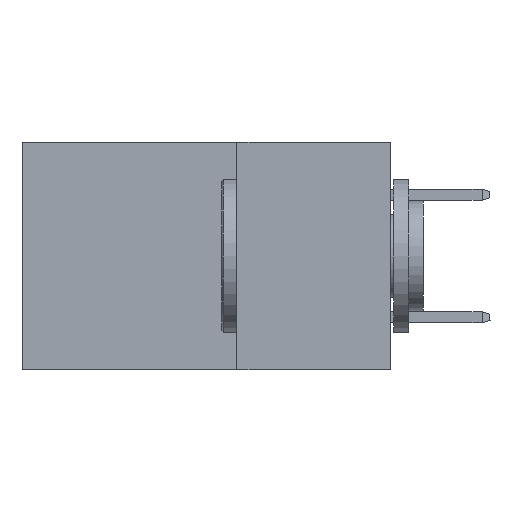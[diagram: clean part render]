
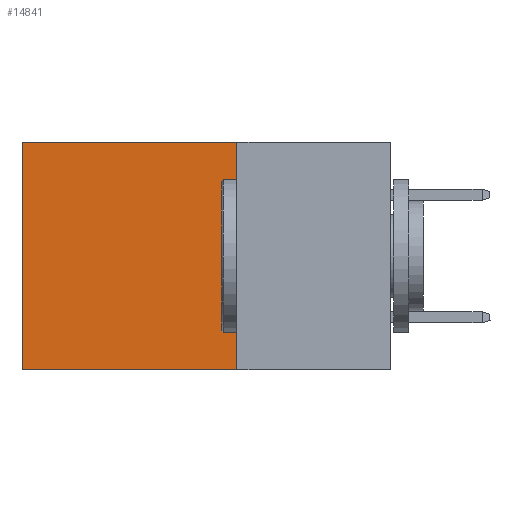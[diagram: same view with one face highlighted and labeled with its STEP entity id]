
A CAD part, left-side view. The second image highlights one B-rep face of the part: STEP entity #14841.
In plain terms, the highlighted planar face has unit normal (-1, 0, 0).
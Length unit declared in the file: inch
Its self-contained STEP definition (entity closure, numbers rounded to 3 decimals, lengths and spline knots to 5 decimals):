
#1457 = DIRECTION ( 'NONE',  ( 1., 0., 0. ) ) ;
#3225 = CARTESIAN_POINT ( 'NONE',  ( 0.2875, 0.25, -0.37 ) ) ;
#3735 = CARTESIAN_POINT ( 'NONE',  ( 0.2875, 0.25, 0. ) ) ;
#4620 = AXIS2_PLACEMENT_3D ( 'NONE', #17867, #1457, #20649 ) ;
#5412 = CARTESIAN_POINT ( 'NONE',  ( 0.2875, 0.25, 0. ) ) ;
#7098 = VERTEX_POINT ( 'NONE', #29846 ) ;
#8364 = LINE ( 'NONE', #5412, #22188 ) ;
#8397 = DIRECTION ( 'NONE',  ( 0., 0., -1. ) ) ;
#9053 = LINE ( 'NONE', #3225, #20254 ) ;
#10389 = ORIENTED_EDGE ( 'NONE', *, *, #23916, .F. ) ;
#12477 = EDGE_CURVE ( 'NONE', #31087, #7098, #18816, .T. ) ;
#14841 = ADVANCED_FACE ( 'NONE', ( #27757 ), #28886, .F. ) ;
#17867 = CARTESIAN_POINT ( 'NONE',  ( 0.2875, 0.25, 0. ) ) ;
#18354 = VERTEX_POINT ( 'NONE', #23366 ) ;
#18816 = LINE ( 'NONE', #32471, #34385 ) ;
#20254 = VECTOR ( 'NONE', #33315, 39.37008 ) ;
#20649 = DIRECTION ( 'NONE',  ( 0., 0., -1. ) ) ;
#21237 = EDGE_CURVE ( 'NONE', #31087, #18354, #8364, .T. ) ;
#21810 = EDGE_LOOP ( 'NONE', ( #23394, #10389, #23186, #24629 ) ) ;
#22188 = VECTOR ( 'NONE', #8397, 39.37008 ) ;
#23186 = ORIENTED_EDGE ( 'NONE', *, *, #21237, .F. ) ;
#23366 = CARTESIAN_POINT ( 'NONE',  ( 0.2875, 0.25, -0.37 ) ) ;
#23394 = ORIENTED_EDGE ( 'NONE', *, *, #24136, .T. ) ;
#23916 = EDGE_CURVE ( 'NONE', #18354, #26583, #9053, .T. ) ;
#24136 = EDGE_CURVE ( 'NONE', #7098, #26583, #25014, .T. ) ;
#24629 = ORIENTED_EDGE ( 'NONE', *, *, #12477, .T. ) ;
#25014 = LINE ( 'NONE', #34627, #33158 ) ;
#26583 = VERTEX_POINT ( 'NONE', #32573 ) ;
#27757 = FACE_OUTER_BOUND ( 'NONE', #21810, .T. ) ;
#28886 = PLANE ( 'NONE',  #4620 ) ;
#29323 = DIRECTION ( 'NONE',  ( 0., 0., -1. ) ) ;
#29846 = CARTESIAN_POINT ( 'NONE',  ( 0.2875, 0.6, 0. ) ) ;
#31087 = VERTEX_POINT ( 'NONE', #3735 ) ;
#32471 = CARTESIAN_POINT ( 'NONE',  ( 0.2875, 0.25, 0. ) ) ;
#32573 = CARTESIAN_POINT ( 'NONE',  ( 0.2875, 0.6, -0.37 ) ) ;
#33158 = VECTOR ( 'NONE', #29323, 39.37008 ) ;
#33315 = DIRECTION ( 'NONE',  ( 0., 1., 0. ) ) ;
#34385 = VECTOR ( 'NONE', #35122, 39.37008 ) ;
#34627 = CARTESIAN_POINT ( 'NONE',  ( 0.2875, 0.6, 0. ) ) ;
#35122 = DIRECTION ( 'NONE',  ( 0., 1., 0. ) ) ;
